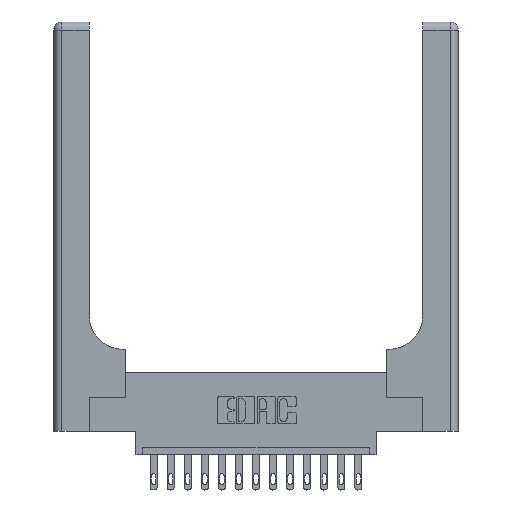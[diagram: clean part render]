
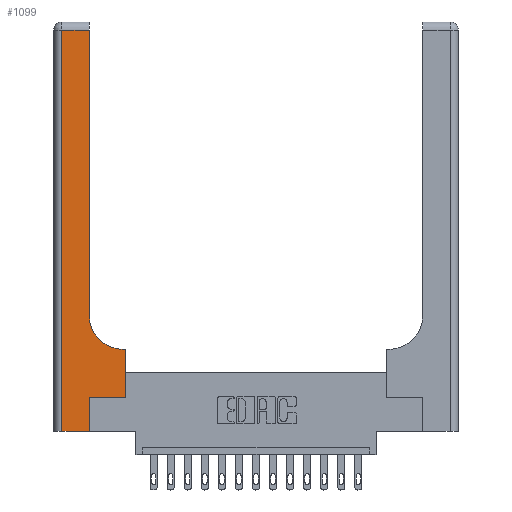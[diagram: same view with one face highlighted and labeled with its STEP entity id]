
A CAD part, top view. The second image highlights one B-rep face of the part: STEP entity #1099.
In plain terms, the highlighted planar face has unit normal (0, 0, 1).
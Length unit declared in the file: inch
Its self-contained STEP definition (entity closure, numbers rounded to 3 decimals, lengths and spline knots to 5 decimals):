
#18 = FACE_OUTER_BOUND ( 'NONE', #14101, .T. ) ;
#180 = ORIENTED_EDGE ( 'NONE', *, *, #17600, .T. ) ;
#610 = LINE ( 'NONE', #15682, #7806 ) ;
#768 = CARTESIAN_POINT ( 'NONE',  ( 0.265, 0., 0.37 ) ) ;
#843 = LINE ( 'NONE', #4952, #3204 ) ;
#901 = VERTEX_POINT ( 'NONE', #8290 ) ;
#948 = DIRECTION ( 'NONE',  ( 1., 0., 0. ) ) ;
#952 = LINE ( 'NONE', #6658, #2948 ) ;
#998 = VERTEX_POINT ( 'NONE', #3275 ) ;
#1099 = ADVANCED_FACE ( 'NONE', ( #18 ), #17615, .F. ) ;
#1559 = EDGE_CURVE ( 'NONE', #13140, #15750, #9804, .T. ) ;
#1640 = DIRECTION ( 'NONE',  ( -1., 0., 0. ) ) ;
#2603 = DIRECTION ( 'NONE',  ( 0., 1., 0. ) ) ;
#2630 = VECTOR ( 'NONE', #11326, 39.37008 ) ;
#2855 = ORIENTED_EDGE ( 'NONE', *, *, #11038, .T. ) ;
#2948 = VECTOR ( 'NONE', #12040, 39.37008 ) ;
#3068 = CARTESIAN_POINT ( 'NONE',  ( 0.51, 0.6, 0.37 ) ) ;
#3204 = VECTOR ( 'NONE', #9322, 39.37008 ) ;
#3207 = CARTESIAN_POINT ( 'NONE',  ( 0.51, 0.85, 0.37 ) ) ;
#3275 = CARTESIAN_POINT ( 'NONE',  ( 0.06, 2.94, 0.37 ) ) ;
#3666 = CARTESIAN_POINT ( 'NONE',  ( 0.528, 0.25, 0.37 ) ) ;
#3800 = VECTOR ( 'NONE', #16766, 39.37008 ) ;
#3937 = CARTESIAN_POINT ( 'NONE',  ( 0.265, 0., 0.37 ) ) ;
#4526 = CARTESIAN_POINT ( 'NONE',  ( 0.26, 3., 0.37 ) ) ;
#4952 = CARTESIAN_POINT ( 'NONE',  ( 0.06, 3., 0.37 ) ) ;
#5131 = EDGE_CURVE ( 'NONE', #6887, #6788, #952, .T. ) ;
#5233 = VERTEX_POINT ( 'NONE', #13532 ) ;
#5469 = CARTESIAN_POINT ( 'NONE',  ( 0., 3., 0.37 ) ) ;
#5778 = ORIENTED_EDGE ( 'NONE', *, *, #1559, .T. ) ;
#5886 = CARTESIAN_POINT ( 'NONE',  ( 0.26, 2.94, 0.37 ) ) ;
#6401 = VECTOR ( 'NONE', #10448, 39.37008 ) ;
#6436 = DIRECTION ( 'NONE',  ( 0., 1., 0. ) ) ;
#6658 = CARTESIAN_POINT ( 'NONE',  ( 0.26, 0.6, 0.37 ) ) ;
#6788 = VERTEX_POINT ( 'NONE', #3068 ) ;
#6887 = VERTEX_POINT ( 'NONE', #10287 ) ;
#7003 = CIRCLE ( 'NONE', #9297, 0.25 ) ;
#7042 = DIRECTION ( 'NONE',  ( 1., 0., 0. ) ) ;
#7789 = LINE ( 'NONE', #3937, #13791 ) ;
#7806 = VECTOR ( 'NONE', #948, 39.37008 ) ;
#8109 = LINE ( 'NONE', #4526, #2630 ) ;
#8290 = CARTESIAN_POINT ( 'NONE',  ( 0.528, 0.25, 0.37 ) ) ;
#8347 = DIRECTION ( 'NONE',  ( 0., 0., -1. ) ) ;
#8402 = DIRECTION ( 'NONE',  ( 0., 0., -1. ) ) ;
#8416 = VERTEX_POINT ( 'NONE', #9231 ) ;
#9231 = CARTESIAN_POINT ( 'NONE',  ( 0.265, 0.25, 0.37 ) ) ;
#9297 = AXIS2_PLACEMENT_3D ( 'NONE', #3207, #8402, #7042 ) ;
#9322 = DIRECTION ( 'NONE',  ( 0., -1., 0. ) ) ;
#9410 = EDGE_CURVE ( 'NONE', #5233, #15211, #8109, .T. ) ;
#9804 = LINE ( 'NONE', #16676, #3800 ) ;
#10287 = CARTESIAN_POINT ( 'NONE',  ( 0.528, 0.6, 0.37 ) ) ;
#10448 = DIRECTION ( 'NONE',  ( -1., 0., 0. ) ) ;
#10455 = LINE ( 'NONE', #3666, #14418 ) ;
#10647 = ORIENTED_EDGE ( 'NONE', *, *, #13346, .T. ) ;
#10711 = LINE ( 'NONE', #17221, #6401 ) ;
#11038 = EDGE_CURVE ( 'NONE', #998, #13140, #843, .T. ) ;
#11122 = ORIENTED_EDGE ( 'NONE', *, *, #17335, .T. ) ;
#11326 = DIRECTION ( 'NONE',  ( 0., 1., 0. ) ) ;
#11973 = AXIS2_PLACEMENT_3D ( 'NONE', #5469, #8347, #1640 ) ;
#12040 = DIRECTION ( 'NONE',  ( -1., 0., 0. ) ) ;
#12341 = EDGE_CURVE ( 'NONE', #8416, #901, #610, .T. ) ;
#12760 = ORIENTED_EDGE ( 'NONE', *, *, #12341, .T. ) ;
#13140 = VERTEX_POINT ( 'NONE', #17066 ) ;
#13346 = EDGE_CURVE ( 'NONE', #15750, #8416, #7789, .T. ) ;
#13532 = CARTESIAN_POINT ( 'NONE',  ( 0.26, 0.85, 0.37 ) ) ;
#13613 = ORIENTED_EDGE ( 'NONE', *, *, #9410, .T. ) ;
#13684 = EDGE_CURVE ( 'NONE', #15211, #998, #10711, .T. ) ;
#13791 = VECTOR ( 'NONE', #2603, 39.37008 ) ;
#14101 = EDGE_LOOP ( 'NONE', ( #13613, #15409, #2855, #5778, #10647, #12760, #11122, #16517, #180 ) ) ;
#14418 = VECTOR ( 'NONE', #6436, 39.37008 ) ;
#15211 = VERTEX_POINT ( 'NONE', #5886 ) ;
#15409 = ORIENTED_EDGE ( 'NONE', *, *, #13684, .T. ) ;
#15682 = CARTESIAN_POINT ( 'NONE',  ( 0.265, 0.25, 0.37 ) ) ;
#15750 = VERTEX_POINT ( 'NONE', #768 ) ;
#16517 = ORIENTED_EDGE ( 'NONE', *, *, #5131, .T. ) ;
#16676 = CARTESIAN_POINT ( 'NONE',  ( 0., 0., 0.37 ) ) ;
#16766 = DIRECTION ( 'NONE',  ( 1., 0., 0. ) ) ;
#17066 = CARTESIAN_POINT ( 'NONE',  ( 0.06, 0., 0.37 ) ) ;
#17221 = CARTESIAN_POINT ( 'NONE',  ( 0., 2.94, 0.37 ) ) ;
#17335 = EDGE_CURVE ( 'NONE', #901, #6887, #10455, .T. ) ;
#17600 = EDGE_CURVE ( 'NONE', #6788, #5233, #7003, .T. ) ;
#17615 = PLANE ( 'NONE',  #11973 ) ;
